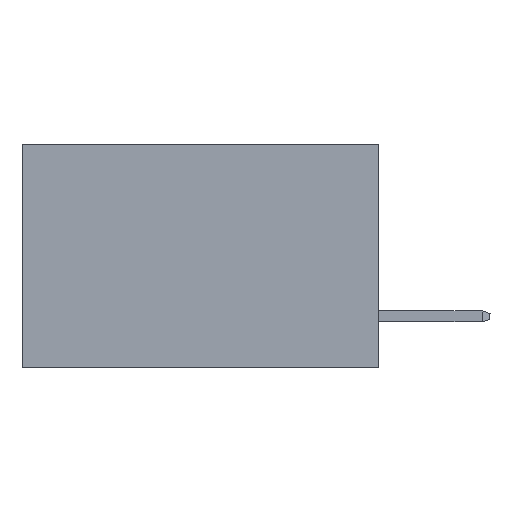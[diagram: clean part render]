
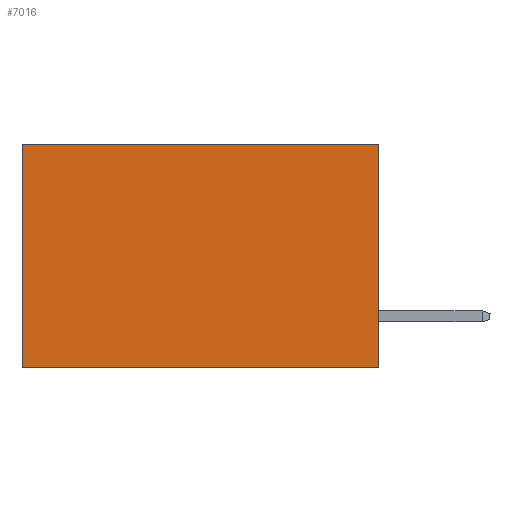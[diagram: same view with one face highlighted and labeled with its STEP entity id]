
A CAD part, left-side view. The second image highlights one B-rep face of the part: STEP entity #7016.
In plain terms, the highlighted planar face has unit normal (-1, 0, 0).
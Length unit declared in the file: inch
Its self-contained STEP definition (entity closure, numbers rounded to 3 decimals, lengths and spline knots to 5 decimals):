
#261 = CARTESIAN_POINT ( 'NONE',  ( 0.277, 0.59, -0.37 ) ) ;
#527 = DIRECTION ( 'NONE',  ( 0., 0., -1. ) ) ;
#864 = VECTOR ( 'NONE', #8623, 39.37008 ) ;
#930 = AXIS2_PLACEMENT_3D ( 'NONE', #9032, #8189, #3004 ) ;
#3004 = DIRECTION ( 'NONE',  ( 0., 0., -1. ) ) ;
#3049 = ORIENTED_EDGE ( 'NONE', *, *, #7530, .T. ) ;
#3142 = LINE ( 'NONE', #10302, #7719 ) ;
#3638 = EDGE_LOOP ( 'NONE', ( #11153, #8738, #9882, #3049 ) ) ;
#4434 = DIRECTION ( 'NONE',  ( 0., 1., 0. ) ) ;
#4636 = LINE ( 'NONE', #261, #10993 ) ;
#4750 = VERTEX_POINT ( 'NONE', #9197 ) ;
#5243 = DIRECTION ( 'NONE',  ( 0., 1., 0. ) ) ;
#5285 = VECTOR ( 'NONE', #5243, 39.37008 ) ;
#5983 = VERTEX_POINT ( 'NONE', #6060 ) ;
#6060 = CARTESIAN_POINT ( 'NONE',  ( 0.277, 0.59, 0. ) ) ;
#6097 = EDGE_CURVE ( 'NONE', #6132, #4750, #10289, .T. ) ;
#6132 = VERTEX_POINT ( 'NONE', #10801 ) ;
#6440 = PLANE ( 'NONE',  #930 ) ;
#6821 = EDGE_CURVE ( 'NONE', #5983, #8759, #4636, .T. ) ;
#7016 = ADVANCED_FACE ( 'NONE', ( #7516 ), #6440, .F. ) ;
#7508 = LINE ( 'NONE', #8719, #5285 ) ;
#7516 = FACE_OUTER_BOUND ( 'NONE', #3638, .T. ) ;
#7530 = EDGE_CURVE ( 'NONE', #6132, #5983, #7508, .T. ) ;
#7719 = VECTOR ( 'NONE', #4434, 39.37008 ) ;
#8189 = DIRECTION ( 'NONE',  ( 1., 0., 0. ) ) ;
#8623 = DIRECTION ( 'NONE',  ( 0., 0., -1. ) ) ;
#8719 = CARTESIAN_POINT ( 'NONE',  ( 0.277, 0., 0. ) ) ;
#8738 = ORIENTED_EDGE ( 'NONE', *, *, #10702, .F. ) ;
#8759 = VERTEX_POINT ( 'NONE', #10835 ) ;
#9032 = CARTESIAN_POINT ( 'NONE',  ( 0.277, 0., -0.37 ) ) ;
#9197 = CARTESIAN_POINT ( 'NONE',  ( 0.277, 0., -0.37 ) ) ;
#9882 = ORIENTED_EDGE ( 'NONE', *, *, #6097, .F. ) ;
#10289 = LINE ( 'NONE', #10720, #864 ) ;
#10302 = CARTESIAN_POINT ( 'NONE',  ( 0.277, 0., -0.37 ) ) ;
#10702 = EDGE_CURVE ( 'NONE', #4750, #8759, #3142, .T. ) ;
#10720 = CARTESIAN_POINT ( 'NONE',  ( 0.277, 0., -0.37 ) ) ;
#10801 = CARTESIAN_POINT ( 'NONE',  ( 0.277, 0., 0. ) ) ;
#10835 = CARTESIAN_POINT ( 'NONE',  ( 0.277, 0.59, -0.37 ) ) ;
#10993 = VECTOR ( 'NONE', #527, 39.37008 ) ;
#11153 = ORIENTED_EDGE ( 'NONE', *, *, #6821, .T. ) ;
